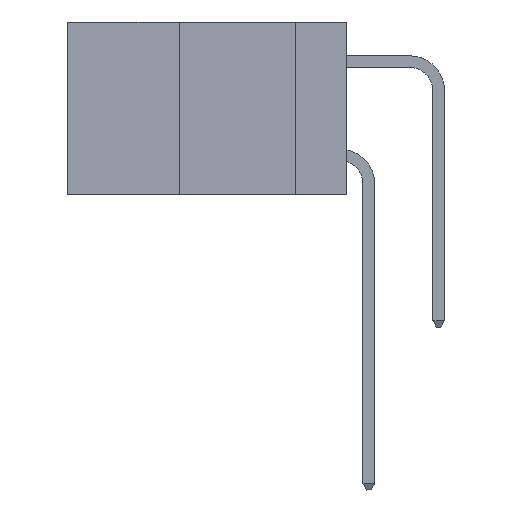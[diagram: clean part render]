
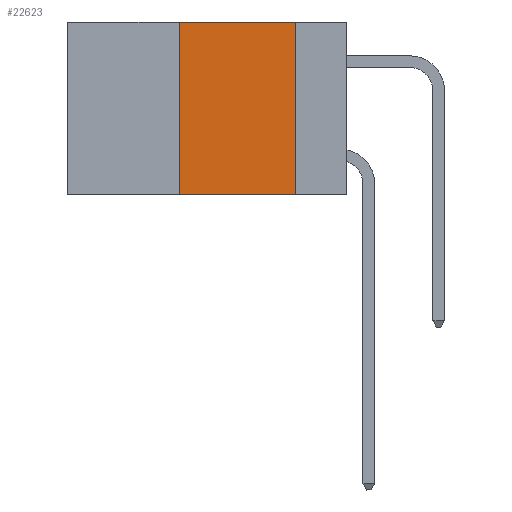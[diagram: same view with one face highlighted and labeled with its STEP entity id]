
A CAD part, left-side view. The second image highlights one B-rep face of the part: STEP entity #22623.
In plain terms, the highlighted planar face has unit normal (-1, 0, 0).
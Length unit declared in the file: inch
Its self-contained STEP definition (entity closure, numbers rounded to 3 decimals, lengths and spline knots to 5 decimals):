
#1087 = CARTESIAN_POINT ( 'NONE',  ( 0., 0.36, 0. ) ) ;
#1442 = VECTOR ( 'NONE', #25023, 39.37008 ) ;
#1991 = VERTEX_POINT ( 'NONE', #7402 ) ;
#2008 = ORIENTED_EDGE ( 'NONE', *, *, #11624, .T. ) ;
#2075 = CARTESIAN_POINT ( 'NONE',  ( 0., 0.6, 0. ) ) ;
#2210 = DIRECTION ( 'NONE',  ( 0., -1., 0. ) ) ;
#2239 = VECTOR ( 'NONE', #7506, 39.37008 ) ;
#2293 = CARTESIAN_POINT ( 'NONE',  ( 0., 0.36, -0.37 ) ) ;
#3324 = EDGE_CURVE ( 'NONE', #15441, #26308, #25237, .T. ) ;
#5493 = VECTOR ( 'NONE', #21012, 39.37008 ) ;
#5527 = CARTESIAN_POINT ( 'NONE',  ( 0., 0.6, 0. ) ) ;
#6158 = DIRECTION ( 'NONE',  ( 0., 0., -1. ) ) ;
#6666 = FACE_OUTER_BOUND ( 'NONE', #10852, .T. ) ;
#7402 = CARTESIAN_POINT ( 'NONE',  ( 0., 0.11, -0.37 ) ) ;
#7506 = DIRECTION ( 'NONE',  ( 0., 0., 1. ) ) ;
#10790 = LINE ( 'NONE', #5527, #1442 ) ;
#10852 = EDGE_LOOP ( 'NONE', ( #19293, #20493, #19021, #2008 ) ) ;
#11624 = EDGE_CURVE ( 'NONE', #15441, #1991, #18473, .T. ) ;
#12447 = CARTESIAN_POINT ( 'NONE',  ( 0., 0.11, 0. ) ) ;
#12513 = LINE ( 'NONE', #12447, #5493 ) ;
#15441 = VERTEX_POINT ( 'NONE', #2293 ) ;
#16502 = CARTESIAN_POINT ( 'NONE',  ( 0., 0.11, 0. ) ) ;
#18473 = LINE ( 'NONE', #24953, #19122 ) ;
#18935 = DIRECTION ( 'NONE',  ( 1., 0., 0. ) ) ;
#19021 = ORIENTED_EDGE ( 'NONE', *, *, #3324, .F. ) ;
#19122 = VECTOR ( 'NONE', #2210, 39.37008 ) ;
#19293 = ORIENTED_EDGE ( 'NONE', *, *, #19348, .F. ) ;
#19309 = AXIS2_PLACEMENT_3D ( 'NONE', #2075, #18935, #6158 ) ;
#19348 = EDGE_CURVE ( 'NONE', #25867, #1991, #12513, .T. ) ;
#20493 = ORIENTED_EDGE ( 'NONE', *, *, #26284, .F. ) ;
#21012 = DIRECTION ( 'NONE',  ( 0., 0., -1. ) ) ;
#22623 = ADVANCED_FACE ( 'NONE', ( #6666 ), #25110, .F. ) ;
#24953 = CARTESIAN_POINT ( 'NONE',  ( 0., 0.6, -0.37 ) ) ;
#25023 = DIRECTION ( 'NONE',  ( 0., -1., 0. ) ) ;
#25110 = PLANE ( 'NONE',  #19309 ) ;
#25237 = LINE ( 'NONE', #1087, #2239 ) ;
#25867 = VERTEX_POINT ( 'NONE', #16502 ) ;
#26284 = EDGE_CURVE ( 'NONE', #26308, #25867, #10790, .T. ) ;
#26308 = VERTEX_POINT ( 'NONE', #27160 ) ;
#27160 = CARTESIAN_POINT ( 'NONE',  ( 0., 0.36, 0. ) ) ;
